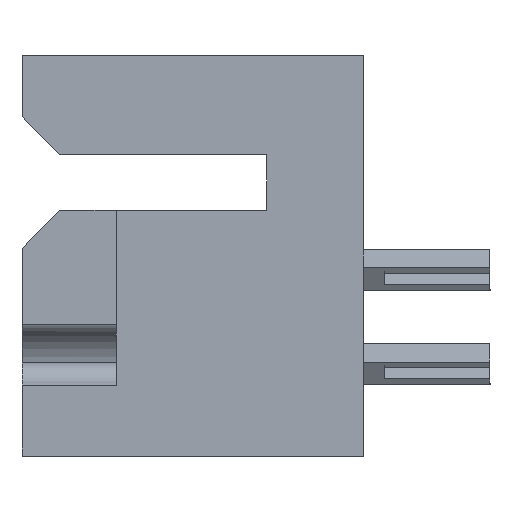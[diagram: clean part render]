
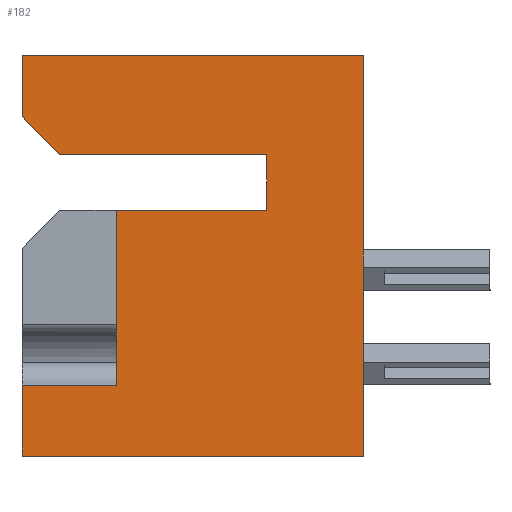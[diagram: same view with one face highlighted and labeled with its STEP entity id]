
A CAD part, left-side view. The second image highlights one B-rep face of the part: STEP entity #182.
In plain terms, the highlighted planar face has unit normal (-1, 0, 0).
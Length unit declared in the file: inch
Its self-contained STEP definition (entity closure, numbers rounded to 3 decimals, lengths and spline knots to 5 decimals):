
#148 = EDGE_CURVE ( 'NONE', #15898, #9324, #16435, .T. ) ;
#182 = ADVANCED_FACE ( 'NONE', ( #2814 ), #3705, .F. ) ;
#542 = VERTEX_POINT ( 'NONE', #11796 ) ;
#674 = CARTESIAN_POINT ( 'NONE',  ( 0., 0.128, -0.131 ) ) ;
#697 = DIRECTION ( 'NONE',  ( 0., 0., 1. ) ) ;
#1045 = DIRECTION ( 'NONE',  ( 0., -1., 0. ) ) ;
#1052 = ORIENTED_EDGE ( 'NONE', *, *, #10393, .F. ) ;
#1445 = VERTEX_POINT ( 'NONE', #2256 ) ;
#1477 = ORIENTED_EDGE ( 'NONE', *, *, #9011, .F. ) ;
#1758 = CARTESIAN_POINT ( 'NONE',  ( 0., 0.328, -0.205 ) ) ;
#1790 = DIRECTION ( 'NONE',  ( 0., 0., 1. ) ) ;
#1830 = DIRECTION ( 'NONE',  ( 0., 0., 1. ) ) ;
#2256 = CARTESIAN_POINT ( 'NONE',  ( 0., 0.128, -0.131 ) ) ;
#2814 = FACE_OUTER_BOUND ( 'NONE', #6102, .T. ) ;
#2934 = CARTESIAN_POINT ( 'NONE',  ( 0., 0., 0. ) ) ;
#3011 = EDGE_CURVE ( 'NONE', #4137, #13809, #6679, .T. ) ;
#3326 = CARTESIAN_POINT ( 'NONE',  ( 0., 0.328, -0.437 ) ) ;
#3402 = EDGE_CURVE ( 'NONE', #14909, #9534, #12838, .T. ) ;
#3439 = EDGE_CURVE ( 'NONE', #14909, #9324, #8230, .T. ) ;
#3564 = DIRECTION ( 'NONE',  ( 0., 0., 1. ) ) ;
#3588 = DIRECTION ( 'NONE',  ( 0., 1., 0. ) ) ;
#3705 = PLANE ( 'NONE',  #10301 ) ;
#3837 = EDGE_CURVE ( 'NONE', #5435, #4137, #11620, .T. ) ;
#3843 = DIRECTION ( 'NONE',  ( 0., 1., 0. ) ) ;
#4137 = VERTEX_POINT ( 'NONE', #4417 ) ;
#4417 = CARTESIAN_POINT ( 'NONE',  ( 0., 0., -0.531 ) ) ;
#4433 = ORIENTED_EDGE ( 'NONE', *, *, #3439, .F. ) ;
#4675 = LINE ( 'NONE', #13481, #9514 ) ;
#4904 = ORIENTED_EDGE ( 'NONE', *, *, #19528, .F. ) ;
#4987 = ORIENTED_EDGE ( 'NONE', *, *, #3402, .T. ) ;
#5261 = CARTESIAN_POINT ( 'NONE',  ( 0., 0.453, 0. ) ) ;
#5319 = CARTESIAN_POINT ( 'NONE',  ( 0., 0.453, 0. ) ) ;
#5435 = VERTEX_POINT ( 'NONE', #18153 ) ;
#5526 = LINE ( 'NONE', #674, #8432 ) ;
#5838 = EDGE_CURVE ( 'NONE', #7085, #542, #17576, .T. ) ;
#5856 = ORIENTED_EDGE ( 'NONE', *, *, #148, .T. ) ;
#6102 = EDGE_LOOP ( 'NONE', ( #4987, #1477, #9647, #9164, #4904, #19967, #9310, #7857, #1052, #5856, #4433 ) ) ;
#6663 = DIRECTION ( 'NONE',  ( 0., 1., 0. ) ) ;
#6679 = LINE ( 'NONE', #8446, #11968 ) ;
#7081 = CARTESIAN_POINT ( 'NONE',  ( 0., 0.328, -0.205 ) ) ;
#7085 = VERTEX_POINT ( 'NONE', #9577 ) ;
#7535 = CARTESIAN_POINT ( 'NONE',  ( 0., 0.453, -0.437 ) ) ;
#7801 = LINE ( 'NONE', #14225, #9961 ) ;
#7857 = ORIENTED_EDGE ( 'NONE', *, *, #15142, .F. ) ;
#8176 = DIRECTION ( 'NONE',  ( 0., -0.707, -0.707 ) ) ;
#8230 = LINE ( 'NONE', #1758, #19344 ) ;
#8432 = VECTOR ( 'NONE', #3588, 39.37008 ) ;
#8446 = CARTESIAN_POINT ( 'NONE',  ( 0., 0., 0. ) ) ;
#9011 = EDGE_CURVE ( 'NONE', #5435, #9534, #7801, .T. ) ;
#9115 = CARTESIAN_POINT ( 'NONE',  ( 0., 0.128, -0.205 ) ) ;
#9164 = ORIENTED_EDGE ( 'NONE', *, *, #3011, .T. ) ;
#9310 = ORIENTED_EDGE ( 'NONE', *, *, #5838, .T. ) ;
#9324 = VERTEX_POINT ( 'NONE', #7081 ) ;
#9514 = VECTOR ( 'NONE', #1045, 39.37008 ) ;
#9534 = VERTEX_POINT ( 'NONE', #7535 ) ;
#9577 = CARTESIAN_POINT ( 'NONE',  ( 0., 0.453, -0.081 ) ) ;
#9647 = ORIENTED_EDGE ( 'NONE', *, *, #3837, .T. ) ;
#9961 = VECTOR ( 'NONE', #1790, 39.37008 ) ;
#10301 = AXIS2_PLACEMENT_3D ( 'NONE', #5261, #16027, #17660 ) ;
#10393 = EDGE_CURVE ( 'NONE', #15898, #1445, #14422, .T. ) ;
#10397 = VECTOR ( 'NONE', #12424, 39.37008 ) ;
#10727 = CARTESIAN_POINT ( 'NONE',  ( 0., 0.453, -0.531 ) ) ;
#10990 = EDGE_CURVE ( 'NONE', #7085, #16371, #15344, .T. ) ;
#11149 = VECTOR ( 'NONE', #6663, 39.37008 ) ;
#11544 = VECTOR ( 'NONE', #3843, 39.37008 ) ;
#11620 = LINE ( 'NONE', #10727, #10397 ) ;
#11796 = CARTESIAN_POINT ( 'NONE',  ( 0., 0.403, -0.131 ) ) ;
#11968 = VECTOR ( 'NONE', #14774, 39.37008 ) ;
#12424 = DIRECTION ( 'NONE',  ( 0., -1., 0. ) ) ;
#12838 = LINE ( 'NONE', #3326, #11149 ) ;
#12968 = CARTESIAN_POINT ( 'NONE',  ( 0., 0.128, -0.205 ) ) ;
#13019 = VECTOR ( 'NONE', #8176, 39.37008 ) ;
#13137 = CARTESIAN_POINT ( 'NONE',  ( 0., 0.128, -0.131 ) ) ;
#13481 = CARTESIAN_POINT ( 'NONE',  ( 0., 0.453, 0. ) ) ;
#13809 = VERTEX_POINT ( 'NONE', #2934 ) ;
#13841 = CARTESIAN_POINT ( 'NONE',  ( 0., 0.328, -0.437 ) ) ;
#14225 = CARTESIAN_POINT ( 'NONE',  ( 0., 0.453, 0. ) ) ;
#14244 = CARTESIAN_POINT ( 'NONE',  ( 0., 0.403, -0.131 ) ) ;
#14422 = LINE ( 'NONE', #13137, #17551 ) ;
#14774 = DIRECTION ( 'NONE',  ( 0., 0., 1. ) ) ;
#14909 = VERTEX_POINT ( 'NONE', #13841 ) ;
#15142 = EDGE_CURVE ( 'NONE', #1445, #542, #5526, .T. ) ;
#15344 = LINE ( 'NONE', #5319, #17052 ) ;
#15898 = VERTEX_POINT ( 'NONE', #9115 ) ;
#16027 = DIRECTION ( 'NONE',  ( 1., 0., 0. ) ) ;
#16204 = CARTESIAN_POINT ( 'NONE',  ( 0., 0.453, 0. ) ) ;
#16371 = VERTEX_POINT ( 'NONE', #16204 ) ;
#16435 = LINE ( 'NONE', #12968, #11544 ) ;
#17052 = VECTOR ( 'NONE', #3564, 39.37008 ) ;
#17551 = VECTOR ( 'NONE', #697, 39.37008 ) ;
#17576 = LINE ( 'NONE', #14244, #13019 ) ;
#17660 = DIRECTION ( 'NONE',  ( 0., 0., -1. ) ) ;
#18153 = CARTESIAN_POINT ( 'NONE',  ( 0., 0.453, -0.531 ) ) ;
#19344 = VECTOR ( 'NONE', #1830, 39.37008 ) ;
#19528 = EDGE_CURVE ( 'NONE', #16371, #13809, #4675, .T. ) ;
#19967 = ORIENTED_EDGE ( 'NONE', *, *, #10990, .F. ) ;
